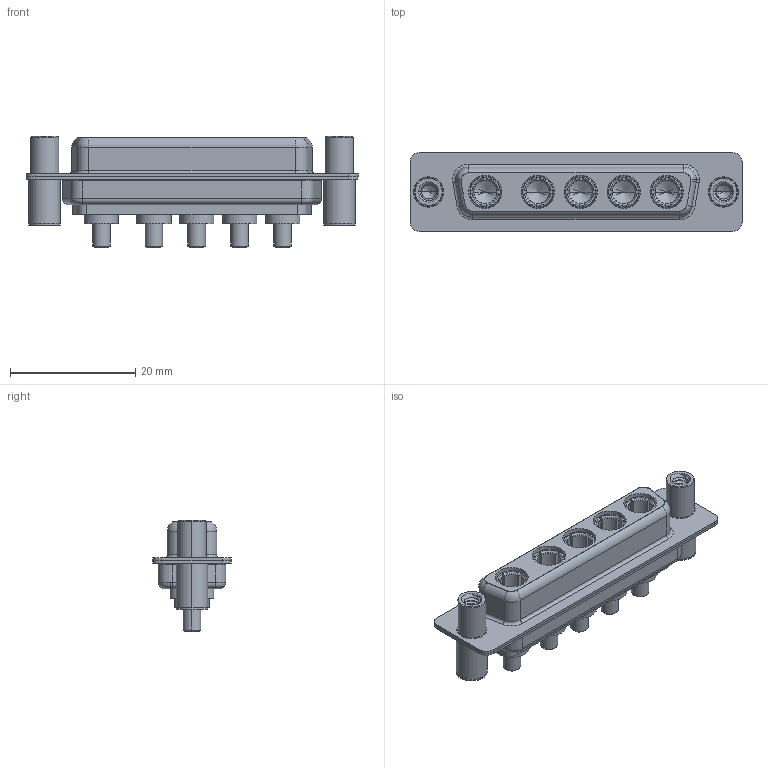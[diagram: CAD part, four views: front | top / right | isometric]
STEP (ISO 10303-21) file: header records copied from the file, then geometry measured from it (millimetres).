
FILE_DESCRIPTION (( 'STEP AP203' ), '1' );
FILE_NAME ('628-5W5-224-2T4.STEP', '2019-05-31T22:34:22', ( '' ), ( '' ), 'SwSTEP 2.0', 'SolidWorks 2016', '' );
FILE_SCHEMA (( 'CONFIG_CONTROL_DESIGN' ));
Length unit declared in the file: millimetre
Products named in the file (6): 628Combo Threaded Standoff and Board Spacer_4; Power Socket_20A S; 628-5W5-224-2T4; 628Combo Housing_5W5; 628Combo Shell Front_25 Contacts; 628Combo Shell Rear_25 Contacts
Assembly tree (10 placements, depth 2):
  628-5W5-224-2T4
    628Combo Housing_5W5
    628Combo Shell Front_25 Contacts
    628Combo Shell Rear_25 Contacts
    628Combo Threaded Standoff and Board Spacer_4  x2
    Power Socket_20A S  x5
Bounding box: 53 x 12.6 x 17.75 mm (x, y, z)
Volume: 4049.3 mm3; surface area: 8818.9 mm2
Topology: 15 solids, 15 shells, 740 faces, 1906 edges, 1210 vertices
Faces by surface type: cylinder 304, plane 218, cone 115, torus 81, bspline 22
Entity records: 14506 total; most frequent: CARTESIAN_POINT 4606, DIRECTION 1981, ORIENTED_EDGE 1912, EDGE_CURVE 956, AXIS2_PLACEMENT_3D 802, VERTEX_POINT 605, EDGE_LOOP 427, CIRCLE 413
